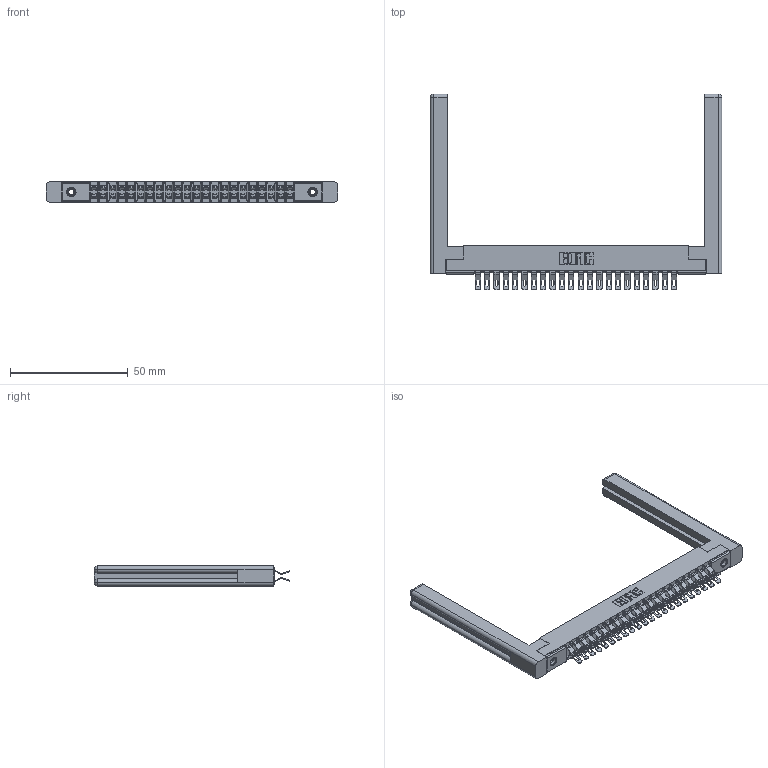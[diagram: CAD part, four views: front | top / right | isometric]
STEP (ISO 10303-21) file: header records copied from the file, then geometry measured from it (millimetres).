
FILE_DESCRIPTION (( 'STEP AP203' ), '1' );
FILE_NAME ('307-044-555-258.STEP', '2019-09-06T07:52:33', ( '' ), ( '' ), 'SwSTEP 2.0', 'SolidWorks 2016', '' );
FILE_SCHEMA (( 'CONFIG_CONTROL_DESIGN' ));
Length unit declared in the file: inch
Products named in the file (5): 307-220-058; 345-250-001_345-250-001-102; 307-044-555-258; 307 Part_.156 Dia Mounting Holes; 307-290-001_555
Assembly tree (49 placements, depth 2):
  307-044-555-258
    307 Part_.156 Dia Mounting Holes
    307-290-001_555  x44
    307-220-058  x2
    345-250-001_345-250-001-102  x2
Bounding box: 123.8 x 83.06 x 8.71 mm (x, y, z)
Volume: 15915.5 mm3; surface area: 20347.8 mm2
Topology: 49 solids, 49 shells, 2967 faces, 8641 edges, 5626 vertices
Faces by surface type: plane 1650, cylinder 1247, sphere 46, torus 12, cone 12
Entity records: 25200 total; most frequent: CARTESIAN_POINT 4153, ORIENTED_EDGE 4058, DIRECTION 4041, EDGE_CURVE 2029, VECTOR 1533, LINE 1533, VERTEX_POINT 1312, AXIS2_PLACEMENT_3D 1254
